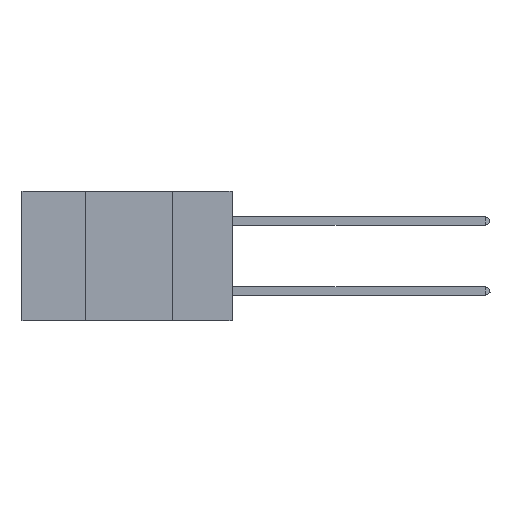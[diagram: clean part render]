
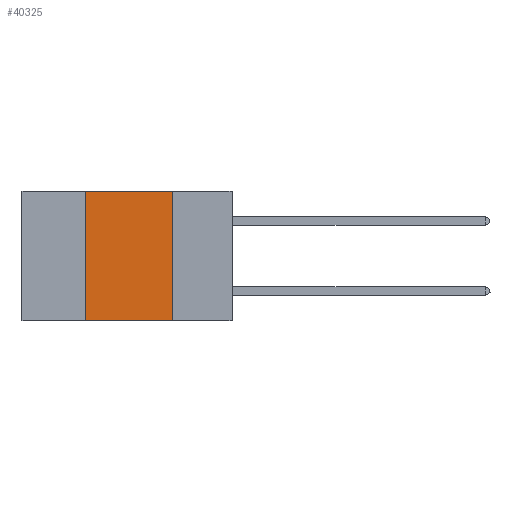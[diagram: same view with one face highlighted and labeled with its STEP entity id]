
A CAD part, left-side view. The second image highlights one B-rep face of the part: STEP entity #40325.
In plain terms, the highlighted planar face has unit normal (-1, 0, 0).
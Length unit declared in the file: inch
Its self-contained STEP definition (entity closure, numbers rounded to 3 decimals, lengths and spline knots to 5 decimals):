
#3695 = CARTESIAN_POINT ( 'NONE',  ( 0., 0.42, -0.37 ) ) ;
#4692 = AXIS2_PLACEMENT_3D ( 'NONE', #5922, #18996, #11700 ) ;
#5922 = CARTESIAN_POINT ( 'NONE',  ( 0., 0.6, 0. ) ) ;
#6315 = VECTOR ( 'NONE', #34592, 39.37008 ) ;
#9716 = CARTESIAN_POINT ( 'NONE',  ( 0., 0.6, -0.37 ) ) ;
#9742 = CARTESIAN_POINT ( 'NONE',  ( 0., 0.42, 0. ) ) ;
#10093 = EDGE_LOOP ( 'NONE', ( #14073, #17435, #19883, #21447 ) ) ;
#11700 = DIRECTION ( 'NONE',  ( 0., 0., -1. ) ) ;
#12200 = VERTEX_POINT ( 'NONE', #18404 ) ;
#14073 = ORIENTED_EDGE ( 'NONE', *, *, #16353, .F. ) ;
#15047 = VERTEX_POINT ( 'NONE', #19680 ) ;
#15114 = LINE ( 'NONE', #42115, #6315 ) ;
#16353 = EDGE_CURVE ( 'NONE', #12200, #41357, #15114, .T. ) ;
#17435 = ORIENTED_EDGE ( 'NONE', *, *, #25915, .F. ) ;
#18404 = CARTESIAN_POINT ( 'NONE',  ( 0., 0.17, 0. ) ) ;
#18564 = PLANE ( 'NONE',  #4692 ) ;
#18996 = DIRECTION ( 'NONE',  ( 1., 0., 0. ) ) ;
#19134 = DIRECTION ( 'NONE',  ( 0., -1., 0. ) ) ;
#19494 = DIRECTION ( 'NONE',  ( 0., 0., 1. ) ) ;
#19680 = CARTESIAN_POINT ( 'NONE',  ( 0., 0.42, 0. ) ) ;
#19883 = ORIENTED_EDGE ( 'NONE', *, *, #35557, .F. ) ;
#20564 = LINE ( 'NONE', #9716, #25087 ) ;
#21447 = ORIENTED_EDGE ( 'NONE', *, *, #36079, .T. ) ;
#22107 = FACE_OUTER_BOUND ( 'NONE', #10093, .T. ) ;
#22232 = VECTOR ( 'NONE', #19134, 39.37008 ) ;
#25087 = VECTOR ( 'NONE', #40500, 39.37008 ) ;
#25915 = EDGE_CURVE ( 'NONE', #15047, #12200, #39285, .T. ) ;
#26785 = CARTESIAN_POINT ( 'NONE',  ( 0., 0.17, -0.37 ) ) ;
#27172 = VECTOR ( 'NONE', #19494, 39.37008 ) ;
#34592 = DIRECTION ( 'NONE',  ( 0., 0., -1. ) ) ;
#34802 = VERTEX_POINT ( 'NONE', #3695 ) ;
#35292 = CARTESIAN_POINT ( 'NONE',  ( 0., 0.6, 0. ) ) ;
#35557 = EDGE_CURVE ( 'NONE', #34802, #15047, #36330, .T. ) ;
#36079 = EDGE_CURVE ( 'NONE', #34802, #41357, #20564, .T. ) ;
#36330 = LINE ( 'NONE', #9742, #27172 ) ;
#39285 = LINE ( 'NONE', #35292, #22232 ) ;
#40325 = ADVANCED_FACE ( 'NONE', ( #22107 ), #18564, .F. ) ;
#40500 = DIRECTION ( 'NONE',  ( 0., -1., 0. ) ) ;
#41357 = VERTEX_POINT ( 'NONE', #26785 ) ;
#42115 = CARTESIAN_POINT ( 'NONE',  ( 0., 0.17, 0. ) ) ;
